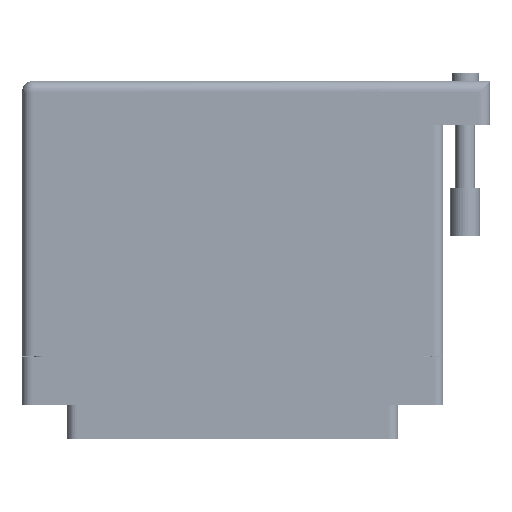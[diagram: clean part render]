
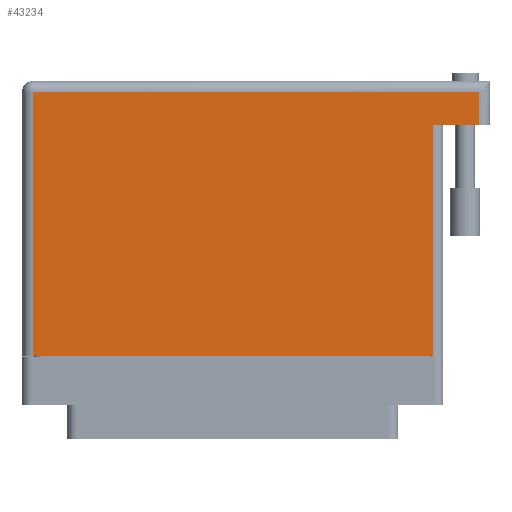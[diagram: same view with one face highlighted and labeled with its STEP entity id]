
A CAD part, front view. The second image highlights one B-rep face of the part: STEP entity #43234.
In plain terms, the highlighted face is planar.
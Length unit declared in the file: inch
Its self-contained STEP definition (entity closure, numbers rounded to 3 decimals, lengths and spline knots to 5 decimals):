
#2808 = VECTOR ( 'NONE', #57414, 39.37008 ) ;
#4886 = CARTESIAN_POINT ( 'NONE',  ( 1.589, 1.675, 0.617 ) ) ;
#6925 = VERTEX_POINT ( 'NONE', #45577 ) ;
#8461 = VERTEX_POINT ( 'NONE', #67985 ) ;
#8831 = LINE ( 'NONE', #58818, #2808 ) ;
#9262 = CARTESIAN_POINT ( 'NONE',  ( 1.589, 1.395, 0.617 ) ) ;
#10444 = VERTEX_POINT ( 'NONE', #57847 ) ;
#10740 = VECTOR ( 'NONE', #21548, 39.37008 ) ;
#11444 = CARTESIAN_POINT ( 'NONE',  ( 1.289, 1.395, 0.617 ) ) ;
#13356 = DIRECTION ( 'NONE',  ( 1., 0., 0. ) ) ;
#15020 = DIRECTION ( 'NONE',  ( -1., 0., 0. ) ) ;
#15516 = VERTEX_POINT ( 'NONE', #22315 ) ;
#19673 = VERTEX_POINT ( 'NONE', #9262 ) ;
#19843 = VECTOR ( 'NONE', #54701, 39.37008 ) ;
#20687 = PLANE ( 'NONE',  #53801 ) ;
#21193 = ORIENTED_EDGE ( 'NONE', *, *, #51651, .T. ) ;
#21548 = DIRECTION ( 'NONE',  ( 0., 1., 0. ) ) ;
#22186 = DIRECTION ( 'NONE',  ( 0., -1., 0. ) ) ;
#22281 = ORIENTED_EDGE ( 'NONE', *, *, #52683, .T. ) ;
#22315 = CARTESIAN_POINT ( 'NONE',  ( -1.289, -0.1, 0.617 ) ) ;
#22456 = CARTESIAN_POINT ( 'NONE',  ( 1.289, -0.1, 0.617 ) ) ;
#26810 = LINE ( 'NONE', #42796, #65293 ) ;
#27028 = CARTESIAN_POINT ( 'NONE',  ( -1.359, 1.675, 0.617 ) ) ;
#29434 = EDGE_CURVE ( 'NONE', #15516, #59417, #40317, .T. ) ;
#34847 = EDGE_CURVE ( 'NONE', #19673, #10444, #35649, .T. ) ;
#35649 = LINE ( 'NONE', #52296, #51421 ) ;
#40317 = LINE ( 'NONE', #41359, #67931 ) ;
#41359 = CARTESIAN_POINT ( 'NONE',  ( -1.359, -0.1, 0.617 ) ) ;
#42327 = DIRECTION ( 'NONE',  ( 0., 0., -1. ) ) ;
#42796 = CARTESIAN_POINT ( 'NONE',  ( -1.289, -0.1, 0.617 ) ) ;
#43234 = ADVANCED_FACE ( 'NONE', ( #52614 ), #20687, .F. ) ;
#43733 = LINE ( 'NONE', #11444, #19843 ) ;
#45577 = CARTESIAN_POINT ( 'NONE',  ( -1.289, 1.605, 0.617 ) ) ;
#47249 = ORIENTED_EDGE ( 'NONE', *, *, #29434, .T. ) ;
#47410 = ORIENTED_EDGE ( 'NONE', *, *, #34847, .F. ) ;
#48438 = ORIENTED_EDGE ( 'NONE', *, *, #51996, .T. ) ;
#49146 = EDGE_LOOP ( 'NONE', ( #47249, #48438, #47410, #21193, #22281, #50271 ) ) ;
#50271 = ORIENTED_EDGE ( 'NONE', *, *, #54665, .T. ) ;
#51421 = VECTOR ( 'NONE', #56927, 39.37008 ) ;
#51651 = EDGE_CURVE ( 'NONE', #19673, #8461, #64818, .T. ) ;
#51996 = EDGE_CURVE ( 'NONE', #59417, #10444, #43733, .T. ) ;
#52296 = CARTESIAN_POINT ( 'NONE',  ( 1.659, 1.395, 0.617 ) ) ;
#52614 = FACE_OUTER_BOUND ( 'NONE', #49146, .T. ) ;
#52683 = EDGE_CURVE ( 'NONE', #8461, #6925, #8831, .T. ) ;
#53801 = AXIS2_PLACEMENT_3D ( 'NONE', #27028, #42327, #15020 ) ;
#54665 = EDGE_CURVE ( 'NONE', #6925, #15516, #26810, .T. ) ;
#54701 = DIRECTION ( 'NONE',  ( 0., 1., 0. ) ) ;
#56927 = DIRECTION ( 'NONE',  ( -1., 0., 0. ) ) ;
#57414 = DIRECTION ( 'NONE',  ( -1., 0., 0. ) ) ;
#57847 = CARTESIAN_POINT ( 'NONE',  ( 1.289, 1.395, 0.617 ) ) ;
#58818 = CARTESIAN_POINT ( 'NONE',  ( -1.359, 1.605, 0.617 ) ) ;
#59417 = VERTEX_POINT ( 'NONE', #22456 ) ;
#64818 = LINE ( 'NONE', #4886, #10740 ) ;
#65293 = VECTOR ( 'NONE', #22186, 39.37008 ) ;
#67931 = VECTOR ( 'NONE', #13356, 39.37008 ) ;
#67985 = CARTESIAN_POINT ( 'NONE',  ( 1.589, 1.605, 0.617 ) ) ;
